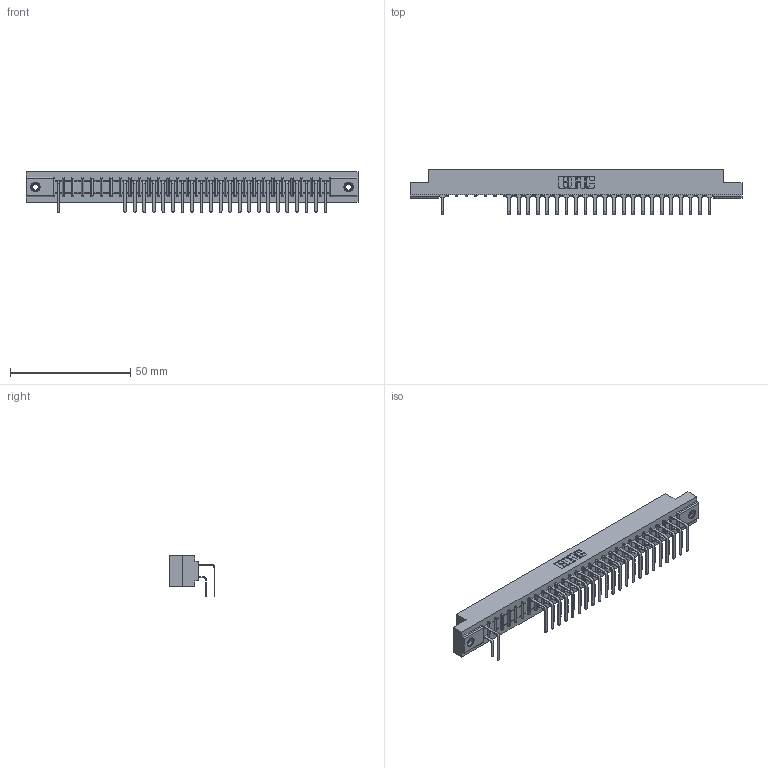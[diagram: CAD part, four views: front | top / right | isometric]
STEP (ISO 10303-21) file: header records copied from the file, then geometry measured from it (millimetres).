
FILE_DESCRIPTION (( 'STEP AP203' ), '1' );
FILE_NAME ('307-058-558-207.STEP', '2018-08-06T07:54:32', ( '' ), ( '' ), 'SwSTEP 2.0', 'SolidWorks 2016', '' );
FILE_SCHEMA (( 'CONFIG_CONTROL_DESIGN' ));
Length unit declared in the file: inch
Products named in the file (5): 307 Part_.156 Dia Mounting Holes; 307-290-001_558 559 - 1 (Single); 307-290-001_558 - 2 (Single); 345-250-001_345-250-005-103; 307-058-558-207
Assembly tree (48 placements, depth 2):
  307-058-558-207
    307 Part_.156 Dia Mounting Holes
    307-290-001_558 559 - 1 (Single)  x22
    307-290-001_558 - 2 (Single)  x23
    345-250-001_345-250-005-103  x2
Bounding box: 137.92 x 18.96 x 16.8 mm (x, y, z)
Volume: 14593.6 mm3; surface area: 17694.7 mm2
Topology: 48 solids, 48 shells, 2588 faces, 7265 edges, 4694 vertices
Faces by surface type: plane 1665, cylinder 847, sphere 60, cone 12, torus 4
Entity records: 29608 total; most frequent: CARTESIAN_POINT 4889, ORIENTED_EDGE 4850, DIRECTION 4789, EDGE_CURVE 2425, VECTOR 1853, LINE 1853, VERTEX_POINT 1568, AXIS2_PLACEMENT_3D 1468
